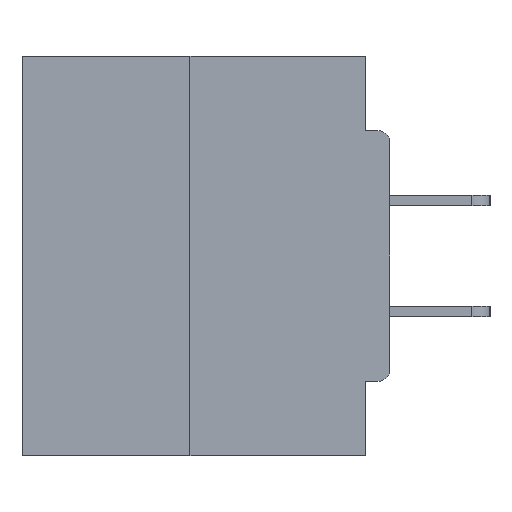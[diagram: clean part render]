
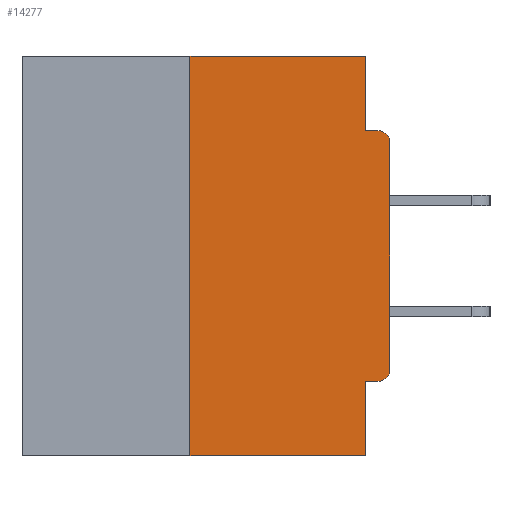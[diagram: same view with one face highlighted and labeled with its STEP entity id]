
A CAD part, left-side view. The second image highlights one B-rep face of the part: STEP entity #14277.
In plain terms, the highlighted planar face has unit normal (-1, 0, 0).
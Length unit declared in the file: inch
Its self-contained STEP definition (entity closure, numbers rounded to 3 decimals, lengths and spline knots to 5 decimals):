
#19 = EDGE_CURVE ( 'NONE', #9980, #26823, #990, .T. ) ;
#126 = LINE ( 'NONE', #5683, #1338 ) ;
#575 = ORIENTED_EDGE ( 'NONE', *, *, #22796, .T. ) ;
#813 = CARTESIAN_POINT ( 'NONE',  ( 0., 0.46, 0. ) ) ;
#990 = LINE ( 'NONE', #813, #13972 ) ;
#996 = DIRECTION ( 'NONE',  ( 0., 1., 0. ) ) ;
#1253 = EDGE_CURVE ( 'NONE', #16022, #13946, #8184, .T. ) ;
#1324 = CARTESIAN_POINT ( 'NONE',  ( 0., 0.25, 0. ) ) ;
#1338 = VECTOR ( 'NONE', #30067, 39.37008 ) ;
#3690 = CARTESIAN_POINT ( 'NONE',  ( 0., 0., -0.4065 ) ) ;
#3793 = CARTESIAN_POINT ( 'NONE',  ( 0., 0.46, 0. ) ) ;
#3795 = EDGE_CURVE ( 'NONE', #16370, #13946, #23866, .T. ) ;
#4132 = PLANE ( 'NONE',  #28099 ) ;
#4516 = EDGE_CURVE ( 'NONE', #32019, #34347, #27741, .T. ) ;
#4873 = DIRECTION ( 'NONE',  ( -1., 0., 0. ) ) ;
#5172 = ORIENTED_EDGE ( 'NONE', *, *, #4516, .F. ) ;
#5683 = CARTESIAN_POINT ( 'NONE',  ( 0., 0.031, 0. ) ) ;
#6193 = DIRECTION ( 'NONE',  ( 0., -1., 0. ) ) ;
#6207 = CARTESIAN_POINT ( 'NONE',  ( 0., 0.46, -0.5 ) ) ;
#6323 = EDGE_CURVE ( 'NONE', #26823, #16370, #126, .T. ) ;
#7932 = ORIENTED_EDGE ( 'NONE', *, *, #10076, .T. ) ;
#8184 = CIRCLE ( 'NONE', #22976, 0.015 ) ;
#8681 = LINE ( 'NONE', #6207, #32673 ) ;
#9527 = CARTESIAN_POINT ( 'NONE',  ( 0., 0., 0. ) ) ;
#9708 = VECTOR ( 'NONE', #26107, 39.37008 ) ;
#9905 = EDGE_LOOP ( 'NONE', ( #34687, #23203, #34733, #16545, #5172, #7932, #575, #19302, #17077, #34633 ) ) ;
#9980 = VERTEX_POINT ( 'NONE', #29902 ) ;
#10076 = EDGE_CURVE ( 'NONE', #32019, #16053, #35128, .T. ) ;
#10236 = CARTESIAN_POINT ( 'NONE',  ( 0., 0.031, -0.5 ) ) ;
#10637 = VECTOR ( 'NONE', #996, 39.37008 ) ;
#11891 = VECTOR ( 'NONE', #12202, 39.37008 ) ;
#12082 = CARTESIAN_POINT ( 'NONE',  ( 0., 0., -0.3915 ) ) ;
#12202 = DIRECTION ( 'NONE',  ( 0., 0., 1. ) ) ;
#12204 = DIRECTION ( 'NONE',  ( 0., 0., 1. ) ) ;
#12226 = DIRECTION ( 'NONE',  ( 0., -1., 0. ) ) ;
#12765 = EDGE_CURVE ( 'NONE', #31421, #13416, #8681, .T. ) ;
#13416 = VERTEX_POINT ( 'NONE', #23060 ) ;
#13946 = VERTEX_POINT ( 'NONE', #22859 ) ;
#13972 = VECTOR ( 'NONE', #6193, 39.37008 ) ;
#14277 = ADVANCED_FACE ( 'NONE', ( #20339 ), #4132, .F. ) ;
#16022 = VERTEX_POINT ( 'NONE', #25989 ) ;
#16053 = VERTEX_POINT ( 'NONE', #12082 ) ;
#16370 = VERTEX_POINT ( 'NONE', #24376 ) ;
#16545 = ORIENTED_EDGE ( 'NONE', *, *, #32229, .F. ) ;
#17077 = ORIENTED_EDGE ( 'NONE', *, *, #3795, .F. ) ;
#17865 = EDGE_CURVE ( 'NONE', #31421, #9980, #27896, .T. ) ;
#18198 = CARTESIAN_POINT ( 'NONE',  ( 0., 0.015, -0.3915 ) ) ;
#19194 = AXIS2_PLACEMENT_3D ( 'NONE', #18198, #4873, #29040 ) ;
#19302 = ORIENTED_EDGE ( 'NONE', *, *, #1253, .T. ) ;
#20339 = FACE_OUTER_BOUND ( 'NONE', #9905, .T. ) ;
#20842 = DIRECTION ( 'NONE',  ( 0., -1., 0. ) ) ;
#21186 = DIRECTION ( 'NONE',  ( -1., 0., 0. ) ) ;
#22485 = DIRECTION ( 'NONE',  ( 1., 0., 0. ) ) ;
#22796 = EDGE_CURVE ( 'NONE', #16053, #16022, #33758, .T. ) ;
#22859 = CARTESIAN_POINT ( 'NONE',  ( 0., 0.015, -0.0935 ) ) ;
#22976 = AXIS2_PLACEMENT_3D ( 'NONE', #24562, #21186, #29919 ) ;
#23060 = CARTESIAN_POINT ( 'NONE',  ( 0., 0.031, -0.5 ) ) ;
#23203 = ORIENTED_EDGE ( 'NONE', *, *, #17865, .F. ) ;
#23866 = LINE ( 'NONE', #31525, #32579 ) ;
#24376 = CARTESIAN_POINT ( 'NONE',  ( 0., 0.031, -0.0935 ) ) ;
#24562 = CARTESIAN_POINT ( 'NONE',  ( 0., 0.015, -0.1085 ) ) ;
#25989 = CARTESIAN_POINT ( 'NONE',  ( 0., 0., -0.1085 ) ) ;
#26107 = DIRECTION ( 'NONE',  ( 0., 0., -1. ) ) ;
#26823 = VERTEX_POINT ( 'NONE', #33196 ) ;
#27741 = LINE ( 'NONE', #3690, #10637 ) ;
#27896 = LINE ( 'NONE', #1324, #31725 ) ;
#27993 = DIRECTION ( 'NONE',  ( 0., 0., -1. ) ) ;
#28099 = AXIS2_PLACEMENT_3D ( 'NONE', #3793, #22485, #27993 ) ;
#29040 = DIRECTION ( 'NONE',  ( 0., 0., -1. ) ) ;
#29413 = CARTESIAN_POINT ( 'NONE',  ( 0., 0.031, -0.4065 ) ) ;
#29902 = CARTESIAN_POINT ( 'NONE',  ( 0., 0.25, 0. ) ) ;
#29919 = DIRECTION ( 'NONE',  ( 0., 0., -1. ) ) ;
#30067 = DIRECTION ( 'NONE',  ( 0., 0., -1. ) ) ;
#30761 = CARTESIAN_POINT ( 'NONE',  ( 0., 0.015, -0.4065 ) ) ;
#31421 = VERTEX_POINT ( 'NONE', #32069 ) ;
#31525 = CARTESIAN_POINT ( 'NONE',  ( 0., 0., -0.0935 ) ) ;
#31725 = VECTOR ( 'NONE', #12204, 39.37008 ) ;
#32019 = VERTEX_POINT ( 'NONE', #30761 ) ;
#32069 = CARTESIAN_POINT ( 'NONE',  ( 0., 0.25, -0.5 ) ) ;
#32229 = EDGE_CURVE ( 'NONE', #34347, #13416, #35016, .T. ) ;
#32579 = VECTOR ( 'NONE', #20842, 39.37008 ) ;
#32673 = VECTOR ( 'NONE', #12226, 39.37008 ) ;
#33196 = CARTESIAN_POINT ( 'NONE',  ( 0., 0.031, 0. ) ) ;
#33758 = LINE ( 'NONE', #9527, #11891 ) ;
#34347 = VERTEX_POINT ( 'NONE', #29413 ) ;
#34633 = ORIENTED_EDGE ( 'NONE', *, *, #6323, .F. ) ;
#34687 = ORIENTED_EDGE ( 'NONE', *, *, #19, .F. ) ;
#34733 = ORIENTED_EDGE ( 'NONE', *, *, #12765, .T. ) ;
#35016 = LINE ( 'NONE', #10236, #9708 ) ;
#35128 = CIRCLE ( 'NONE', #19194, 0.015 ) ;
